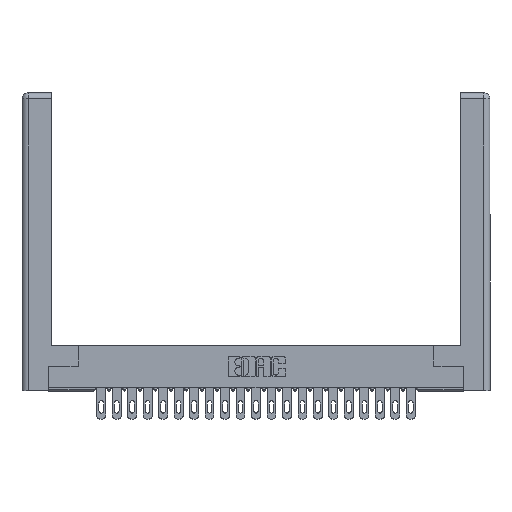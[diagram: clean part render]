
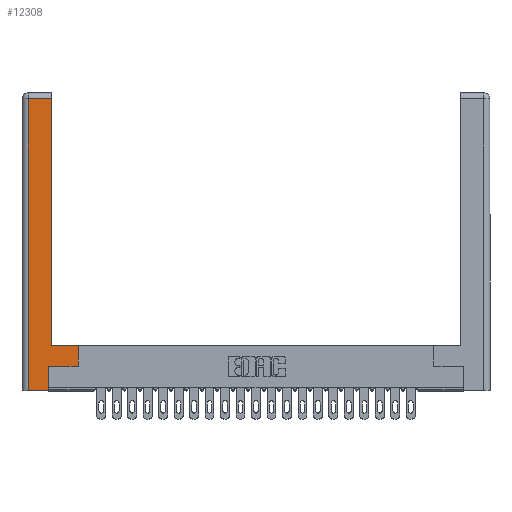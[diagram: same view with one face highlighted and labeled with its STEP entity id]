
A CAD part, top view. The second image highlights one B-rep face of the part: STEP entity #12308.
In plain terms, the highlighted planar face has unit normal (0, 0, 1).
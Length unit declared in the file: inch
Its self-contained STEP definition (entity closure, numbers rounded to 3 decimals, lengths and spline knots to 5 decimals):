
#160 = DIRECTION ( 'NONE',  ( 1., 0., 0. ) ) ;
#340 = CARTESIAN_POINT ( 'NONE',  ( 0.565, 0.245, 0. ) ) ;
#456 = LINE ( 'NONE', #25134, #11919 ) ;
#626 = LINE ( 'NONE', #11384, #1272 ) ;
#1121 = EDGE_CURVE ( 'NONE', #15513, #8659, #5113, .T. ) ;
#1272 = VECTOR ( 'NONE', #2091, 39.37008 ) ;
#1441 = VECTOR ( 'NONE', #20280, 39.37008 ) ;
#1928 = VERTEX_POINT ( 'NONE', #6674 ) ;
#2091 = DIRECTION ( 'NONE',  ( 0., 1., 0. ) ) ;
#2157 = LINE ( 'NONE', #2948, #20698 ) ;
#2202 = ORIENTED_EDGE ( 'NONE', *, *, #13444, .T. ) ;
#2948 = CARTESIAN_POINT ( 'NONE',  ( 0.0615, 0., 0. ) ) ;
#3384 = ORIENTED_EDGE ( 'NONE', *, *, #13862, .T. ) ;
#5113 = LINE ( 'NONE', #17288, #1441 ) ;
#6065 = VERTEX_POINT ( 'NONE', #6888 ) ;
#6674 = CARTESIAN_POINT ( 'NONE',  ( 0.565, 0.245, 0. ) ) ;
#6888 = CARTESIAN_POINT ( 'NONE',  ( 0.565, 0.45, 0. ) ) ;
#6998 = CARTESIAN_POINT ( 'NONE',  ( 0.295, 0.45, 0. ) ) ;
#7018 = CARTESIAN_POINT ( 'NONE',  ( 0.295, 3., 0. ) ) ;
#8659 = VERTEX_POINT ( 'NONE', #13850 ) ;
#8746 = EDGE_CURVE ( 'NONE', #21303, #15904, #456, .T. ) ;
#8910 = ORIENTED_EDGE ( 'NONE', *, *, #8746, .T. ) ;
#9474 = CARTESIAN_POINT ( 'NONE',  ( 0.265, 0., 0. ) ) ;
#9840 = DIRECTION ( 'NONE',  ( 0., 0., -1. ) ) ;
#9901 = AXIS2_PLACEMENT_3D ( 'NONE', #18537, #9840, #25002 ) ;
#11268 = EDGE_CURVE ( 'NONE', #1928, #6065, #626, .T. ) ;
#11343 = CARTESIAN_POINT ( 'NONE',  ( 0.265, 0.245, 0. ) ) ;
#11384 = CARTESIAN_POINT ( 'NONE',  ( 0.565, 0.45, 0. ) ) ;
#11608 = LINE ( 'NONE', #340, #18693 ) ;
#11826 = DIRECTION ( 'NONE',  ( -1., 0., 0. ) ) ;
#11919 = VECTOR ( 'NONE', #12259, 39.37008 ) ;
#12259 = DIRECTION ( 'NONE',  ( 0., 1., 0. ) ) ;
#12308 = ADVANCED_FACE ( 'NONE', ( #15670 ), #22826, .F. ) ;
#13440 = CARTESIAN_POINT ( 'NONE',  ( 0.295, 2.94, 0. ) ) ;
#13444 = EDGE_CURVE ( 'NONE', #6065, #14039, #16640, .T. ) ;
#13529 = CARTESIAN_POINT ( 'NONE',  ( 0.0615, 0., 0. ) ) ;
#13850 = CARTESIAN_POINT ( 'NONE',  ( 0.0615, 2.94, 0. ) ) ;
#13862 = EDGE_CURVE ( 'NONE', #8659, #26353, #2157, .T. ) ;
#14039 = VERTEX_POINT ( 'NONE', #6998 ) ;
#15513 = VERTEX_POINT ( 'NONE', #13440 ) ;
#15670 = FACE_OUTER_BOUND ( 'NONE', #18678, .T. ) ;
#15802 = ORIENTED_EDGE ( 'NONE', *, *, #20124, .T. ) ;
#15904 = VERTEX_POINT ( 'NONE', #11343 ) ;
#16287 = VECTOR ( 'NONE', #26719, 39.37008 ) ;
#16640 = LINE ( 'NONE', #24877, #24461 ) ;
#17288 = CARTESIAN_POINT ( 'NONE',  ( 0.0615, 2.94, 0. ) ) ;
#17982 = LINE ( 'NONE', #9474, #16287 ) ;
#18537 = CARTESIAN_POINT ( 'NONE',  ( 0., 0., 0. ) ) ;
#18652 = ORIENTED_EDGE ( 'NONE', *, *, #11268, .T. ) ;
#18678 = EDGE_LOOP ( 'NONE', ( #26601, #24438, #3384, #26930, #8910, #15802, #18652, #2202 ) ) ;
#18693 = VECTOR ( 'NONE', #160, 39.37008 ) ;
#19617 = EDGE_CURVE ( 'NONE', #14039, #15513, #27888, .T. ) ;
#20124 = EDGE_CURVE ( 'NONE', #15904, #1928, #11608, .T. ) ;
#20280 = DIRECTION ( 'NONE',  ( -1., 0., 0. ) ) ;
#20698 = VECTOR ( 'NONE', #24663, 39.37008 ) ;
#21303 = VERTEX_POINT ( 'NONE', #27841 ) ;
#22826 = PLANE ( 'NONE',  #9901 ) ;
#23510 = VECTOR ( 'NONE', #26325, 39.37008 ) ;
#24004 = EDGE_CURVE ( 'NONE', #26353, #21303, #17982, .T. ) ;
#24438 = ORIENTED_EDGE ( 'NONE', *, *, #1121, .T. ) ;
#24461 = VECTOR ( 'NONE', #11826, 39.37008 ) ;
#24663 = DIRECTION ( 'NONE',  ( 0., -1., 0. ) ) ;
#24877 = CARTESIAN_POINT ( 'NONE',  ( 0.295, 0.45, 0. ) ) ;
#25002 = DIRECTION ( 'NONE',  ( -1., 0., 0. ) ) ;
#25134 = CARTESIAN_POINT ( 'NONE',  ( 0.265, 0.245, 0. ) ) ;
#26325 = DIRECTION ( 'NONE',  ( 0., 1., 0. ) ) ;
#26353 = VERTEX_POINT ( 'NONE', #13529 ) ;
#26601 = ORIENTED_EDGE ( 'NONE', *, *, #19617, .T. ) ;
#26719 = DIRECTION ( 'NONE',  ( 1., 0., 0. ) ) ;
#26930 = ORIENTED_EDGE ( 'NONE', *, *, #24004, .T. ) ;
#27841 = CARTESIAN_POINT ( 'NONE',  ( 0.265, 0., 0. ) ) ;
#27888 = LINE ( 'NONE', #7018, #23510 ) ;
